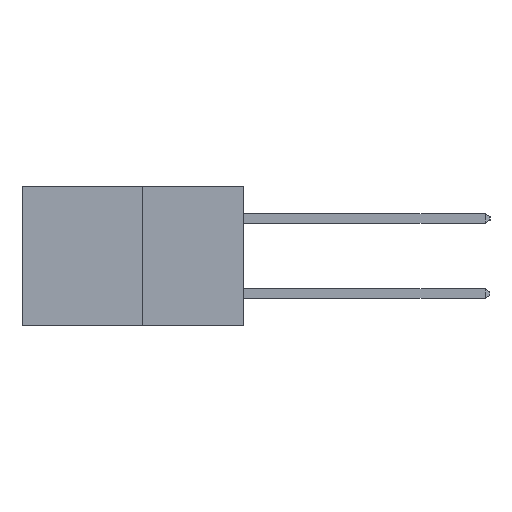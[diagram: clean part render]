
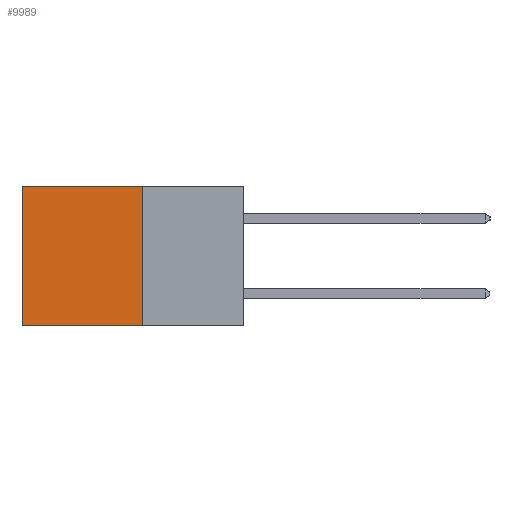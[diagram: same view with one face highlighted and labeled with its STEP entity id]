
A CAD part, left-side view. The second image highlights one B-rep face of the part: STEP entity #9989.
In plain terms, the highlighted planar face has unit normal (-1, 0, 0).
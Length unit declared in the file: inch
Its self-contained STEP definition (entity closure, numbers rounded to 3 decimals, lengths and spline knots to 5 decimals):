
#530 = DIRECTION ( 'NONE',  ( 1., 0., 0. ) ) ;
#934 = LINE ( 'NONE', #15775, #18395 ) ;
#1858 = EDGE_CURVE ( 'NONE', #13081, #4103, #934, .T. ) ;
#2875 = VERTEX_POINT ( 'NONE', #9583 ) ;
#3158 = ORIENTED_EDGE ( 'NONE', *, *, #17093, .F. ) ;
#3454 = FACE_OUTER_BOUND ( 'NONE', #20421, .T. ) ;
#4103 = VERTEX_POINT ( 'NONE', #5806 ) ;
#4143 = CARTESIAN_POINT ( 'NONE',  ( 0.277, 0.27, 0. ) ) ;
#4245 = ORIENTED_EDGE ( 'NONE', *, *, #10129, .F. ) ;
#5092 = VECTOR ( 'NONE', #21016, 39.37008 ) ;
#5093 = ORIENTED_EDGE ( 'NONE', *, *, #1858, .T. ) ;
#5620 = LINE ( 'NONE', #7757, #5092 ) ;
#5806 = CARTESIAN_POINT ( 'NONE',  ( 0.277, 0.59, 0. ) ) ;
#6479 = DIRECTION ( 'NONE',  ( 0., 1., 0. ) ) ;
#7757 = CARTESIAN_POINT ( 'NONE',  ( 0.277, 0.27, -0.37 ) ) ;
#9181 = PLANE ( 'NONE',  #9762 ) ;
#9253 = CARTESIAN_POINT ( 'NONE',  ( 0.277, 0.27, -0.37 ) ) ;
#9583 = CARTESIAN_POINT ( 'NONE',  ( 0.277, 0.59, -0.37 ) ) ;
#9762 = AXIS2_PLACEMENT_3D ( 'NONE', #20742, #530, #12531 ) ;
#9989 = ADVANCED_FACE ( 'NONE', ( #3454 ), #9181, .F. ) ;
#10129 = EDGE_CURVE ( 'NONE', #13081, #13870, #5620, .T. ) ;
#10917 = DIRECTION ( 'NONE',  ( 0., 1., 0. ) ) ;
#12106 = LINE ( 'NONE', #15103, #15491 ) ;
#12531 = DIRECTION ( 'NONE',  ( 0., 0., -1. ) ) ;
#12733 = EDGE_CURVE ( 'NONE', #4103, #2875, #12106, .T. ) ;
#13081 = VERTEX_POINT ( 'NONE', #4143 ) ;
#13870 = VERTEX_POINT ( 'NONE', #16394 ) ;
#14009 = LINE ( 'NONE', #9253, #18918 ) ;
#15103 = CARTESIAN_POINT ( 'NONE',  ( 0.277, 0.59, -0.37 ) ) ;
#15491 = VECTOR ( 'NONE', #18347, 39.37008 ) ;
#15771 = ORIENTED_EDGE ( 'NONE', *, *, #12733, .T. ) ;
#15775 = CARTESIAN_POINT ( 'NONE',  ( 0.277, 0.27, 0. ) ) ;
#16394 = CARTESIAN_POINT ( 'NONE',  ( 0.277, 0.27, -0.37 ) ) ;
#17093 = EDGE_CURVE ( 'NONE', #13870, #2875, #14009, .T. ) ;
#18347 = DIRECTION ( 'NONE',  ( 0., 0., -1. ) ) ;
#18395 = VECTOR ( 'NONE', #6479, 39.37008 ) ;
#18918 = VECTOR ( 'NONE', #10917, 39.37008 ) ;
#20421 = EDGE_LOOP ( 'NONE', ( #15771, #3158, #4245, #5093 ) ) ;
#20742 = CARTESIAN_POINT ( 'NONE',  ( 0.277, 0.27, -0.37 ) ) ;
#21016 = DIRECTION ( 'NONE',  ( 0., 0., -1. ) ) ;
